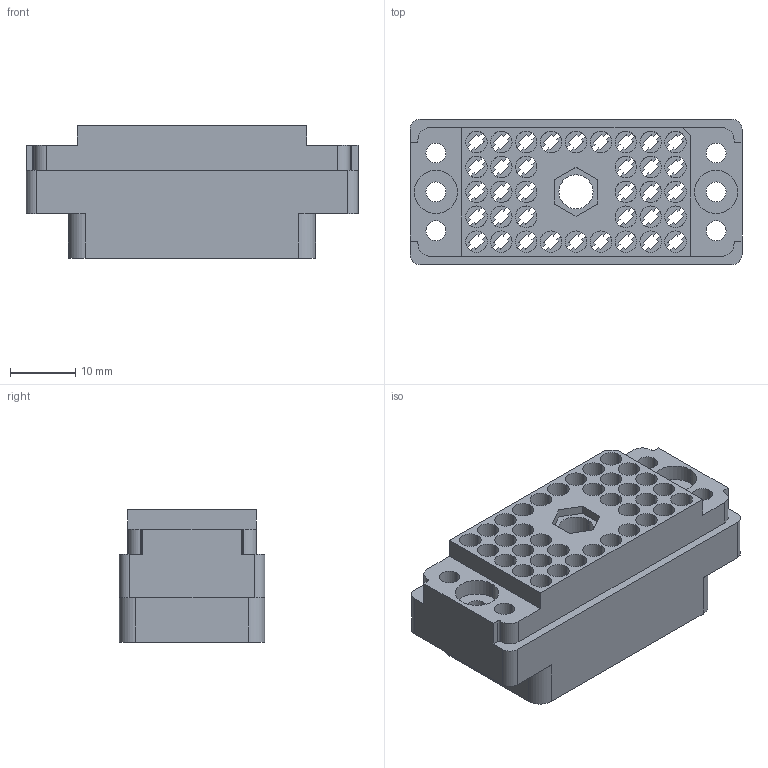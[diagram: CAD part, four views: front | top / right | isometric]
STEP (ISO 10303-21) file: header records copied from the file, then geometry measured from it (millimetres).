
FILE_DESCRIPTION (( 'STEP AP203' ), '1' );
FILE_NAME ('519-036-000-300.STEP', '2020-03-02T21:13:56', ( '' ), ( '' ), 'SwSTEP 2.0', 'SolidWorks 2016', '' );
FILE_SCHEMA (( 'CONFIG_CONTROL_DESIGN' ));
Length unit declared in the file: inch
Products named in the file (2): 519 Plug Insulator_036; 519-036-000-300
Assembly tree (1 placements, depth 2):
  519-036-000-300
    519 Plug Insulator_036
Bounding box: 50.8 x 22.25 x 20.27 mm (x, y, z)
Volume: 8904.2 mm3; surface area: 11386.8 mm2
Topology: 1 solids, 1 shells, 855 faces, 2507 edges, 1670 vertices
Faces by surface type: plane 615, cylinder 238, cone 2
Entity records: 28761 total; most frequent: CARTESIAN_POINT 5036, ORIENTED_EDGE 5014, DIRECTION 4845, EDGE_CURVE 2507, LINE 1887, VECTOR 1887, VERTEX_POINT 1670, AXIS2_PLACEMENT_3D 1479
